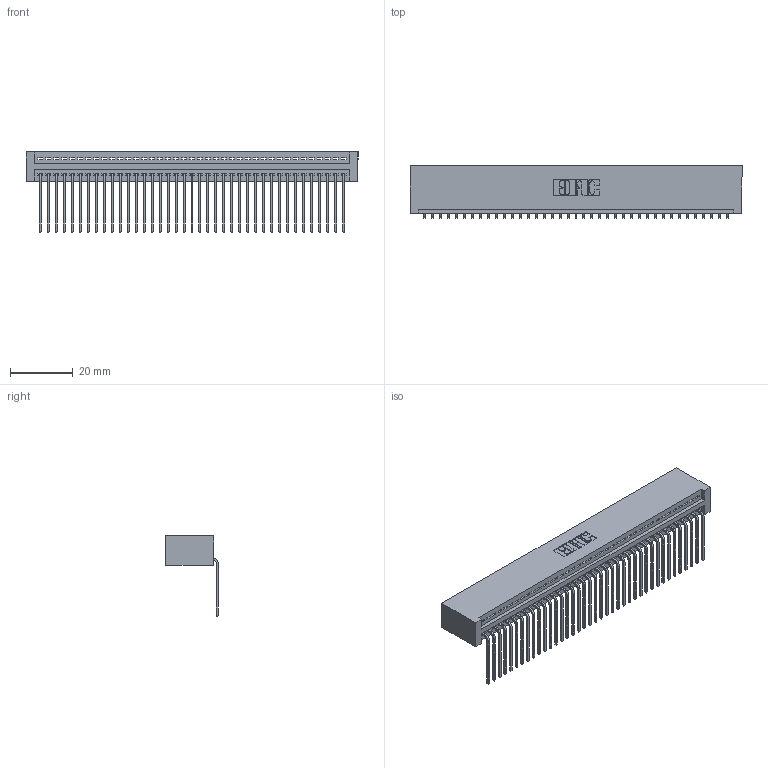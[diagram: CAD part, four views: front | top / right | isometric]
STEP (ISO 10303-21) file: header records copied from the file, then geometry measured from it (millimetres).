
FILE_DESCRIPTION (( 'STEP AP203' ), '1' );
FILE_NAME ('395-039-559-101.STEP', '2018-11-14T14:38:21', ( '' ), ( '' ), 'SwSTEP 2.0', 'SolidWorks 2016', '' );
FILE_SCHEMA (( 'CONFIG_CONTROL_DESIGN' ));
Length unit declared in the file: inch
Products named in the file (3): 345 Part_No Mounting Lugs; 395-039-559-101; 345-292-001_558 559 Tail - 1
Assembly tree (40 placements, depth 2):
  395-039-559-101
    345 Part_No Mounting Lugs
    345-292-001_558 559 Tail - 1  x39
Bounding box: 105.66 x 16.75 x 25.53 mm (x, y, z)
Volume: 10725.8 mm3; surface area: 15166.5 mm2
Topology: 40 solids, 40 shells, 2458 faces, 7415 edges, 4890 vertices
Faces by surface type: plane 1714, cylinder 744
Entity records: 29563 total; most frequent: CARTESIAN_POINT 5129, ORIENTED_EDGE 5102, DIRECTION 4477, EDGE_CURVE 2551, VECTOR 2271, LINE 2271, VERTEX_POINT 1698, AXIS2_PLACEMENT_3D 1103
